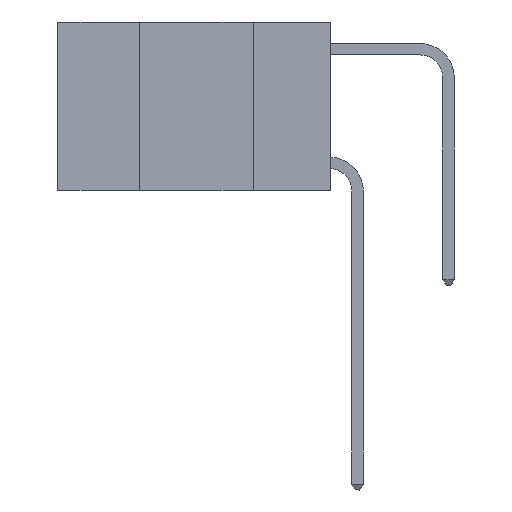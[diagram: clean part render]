
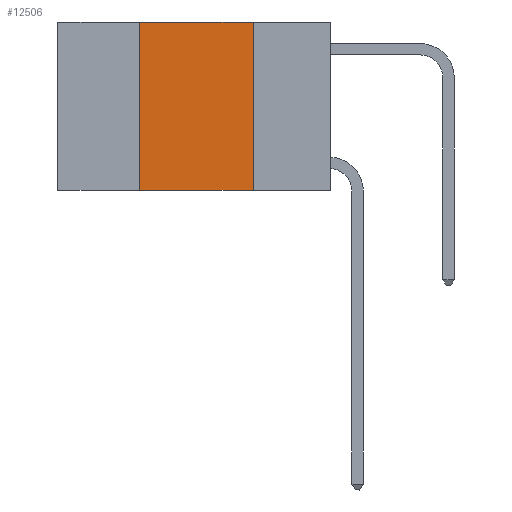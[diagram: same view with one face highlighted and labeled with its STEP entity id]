
A CAD part, left-side view. The second image highlights one B-rep face of the part: STEP entity #12506.
In plain terms, the highlighted planar face has unit normal (-1, 0, 0).
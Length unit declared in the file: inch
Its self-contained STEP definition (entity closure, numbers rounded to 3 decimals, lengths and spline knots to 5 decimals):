
#3 = EDGE_CURVE ( 'NONE', #28051, #24942, #23241, .T. ) ;
#1136 = DIRECTION ( 'NONE',  ( 0., 0., 1. ) ) ;
#1189 = VERTEX_POINT ( 'NONE', #19810 ) ;
#1279 = LINE ( 'NONE', #14106, #12058 ) ;
#2192 = CARTESIAN_POINT ( 'NONE',  ( 0., 0.17, 0. ) ) ;
#2407 = EDGE_LOOP ( 'NONE', ( #11466, #16884, #14641, #19416 ) ) ;
#2634 = EDGE_CURVE ( 'NONE', #20910, #24942, #18998, .T. ) ;
#4416 = CARTESIAN_POINT ( 'NONE',  ( 0., 0.17, -0.37 ) ) ;
#8087 = VECTOR ( 'NONE', #16821, 39.37008 ) ;
#9806 = CARTESIAN_POINT ( 'NONE',  ( 0., 0.6, 0. ) ) ;
#10420 = VECTOR ( 'NONE', #18764, 39.37008 ) ;
#11466 = ORIENTED_EDGE ( 'NONE', *, *, #2634, .F. ) ;
#11812 = LINE ( 'NONE', #9806, #22949 ) ;
#12058 = VECTOR ( 'NONE', #1136, 39.37008 ) ;
#12506 = ADVANCED_FACE ( 'NONE', ( #20963 ), #25433, .F. ) ;
#12848 = CARTESIAN_POINT ( 'NONE',  ( 0., 0.42, -0.37 ) ) ;
#14106 = CARTESIAN_POINT ( 'NONE',  ( 0., 0.42, 0. ) ) ;
#14325 = CARTESIAN_POINT ( 'NONE',  ( 0., 0.6, 0. ) ) ;
#14641 = ORIENTED_EDGE ( 'NONE', *, *, #22762, .F. ) ;
#16789 = EDGE_CURVE ( 'NONE', #1189, #20910, #11812, .T. ) ;
#16821 = DIRECTION ( 'NONE',  ( 0., 0., -1. ) ) ;
#16884 = ORIENTED_EDGE ( 'NONE', *, *, #16789, .F. ) ;
#18629 = CARTESIAN_POINT ( 'NONE',  ( 0., 0.6, -0.37 ) ) ;
#18653 = DIRECTION ( 'NONE',  ( 1., 0., 0. ) ) ;
#18764 = DIRECTION ( 'NONE',  ( 0., -1., 0. ) ) ;
#18998 = LINE ( 'NONE', #23463, #8087 ) ;
#19416 = ORIENTED_EDGE ( 'NONE', *, *, #3, .T. ) ;
#19810 = CARTESIAN_POINT ( 'NONE',  ( 0., 0.42, 0. ) ) ;
#20910 = VERTEX_POINT ( 'NONE', #2192 ) ;
#20963 = FACE_OUTER_BOUND ( 'NONE', #2407, .T. ) ;
#22503 = AXIS2_PLACEMENT_3D ( 'NONE', #14325, #18653, #25294 ) ;
#22762 = EDGE_CURVE ( 'NONE', #28051, #1189, #1279, .T. ) ;
#22949 = VECTOR ( 'NONE', #25375, 39.37008 ) ;
#23241 = LINE ( 'NONE', #18629, #10420 ) ;
#23463 = CARTESIAN_POINT ( 'NONE',  ( 0., 0.17, 0. ) ) ;
#24942 = VERTEX_POINT ( 'NONE', #4416 ) ;
#25294 = DIRECTION ( 'NONE',  ( 0., 0., -1. ) ) ;
#25375 = DIRECTION ( 'NONE',  ( 0., -1., 0. ) ) ;
#25433 = PLANE ( 'NONE',  #22503 ) ;
#28051 = VERTEX_POINT ( 'NONE', #12848 ) ;
